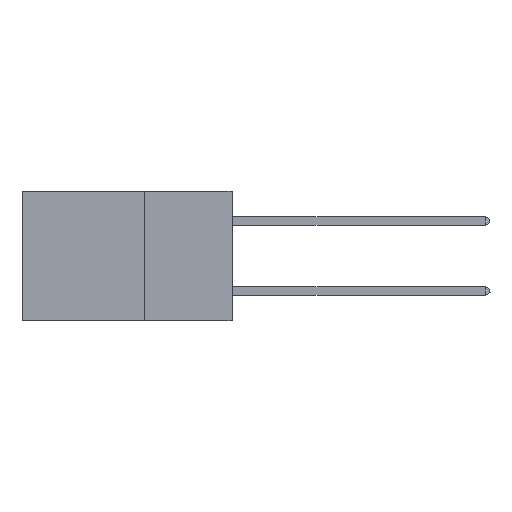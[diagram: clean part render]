
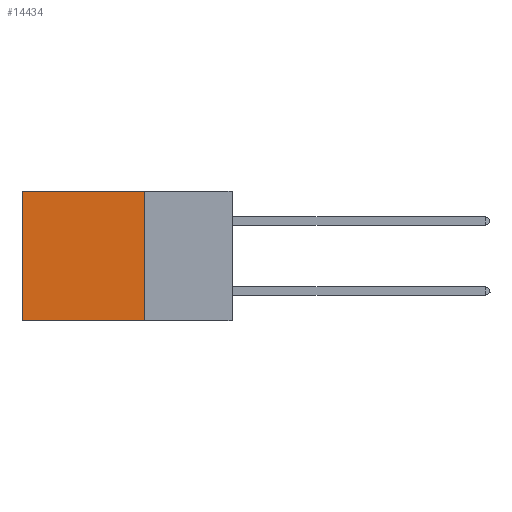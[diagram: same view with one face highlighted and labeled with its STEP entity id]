
A CAD part, left-side view. The second image highlights one B-rep face of the part: STEP entity #14434.
In plain terms, the highlighted planar face has unit normal (-1, 0, 0).
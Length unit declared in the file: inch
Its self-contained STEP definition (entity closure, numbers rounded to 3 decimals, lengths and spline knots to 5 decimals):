
#83 = AXIS2_PLACEMENT_3D ( 'NONE', #19987, #11305, #1250 ) ;
#1067 = EDGE_CURVE ( 'NONE', #20200, #18856, #13007, .T. ) ;
#1250 = DIRECTION ( 'NONE',  ( 0., 0., -1. ) ) ;
#2143 = FACE_OUTER_BOUND ( 'NONE', #9424, .T. ) ;
#2259 = CARTESIAN_POINT ( 'NONE',  ( 0.2875, 0.25, -0.37 ) ) ;
#2414 = CARTESIAN_POINT ( 'NONE',  ( 0.2875, 0.25, 0. ) ) ;
#5028 = VERTEX_POINT ( 'NONE', #18991 ) ;
#6157 = CARTESIAN_POINT ( 'NONE',  ( 0.2875, 0.25, 0. ) ) ;
#6724 = DIRECTION ( 'NONE',  ( 0., 1., 0. ) ) ;
#6842 = EDGE_CURVE ( 'NONE', #18856, #5028, #13062, .T. ) ;
#8876 = VERTEX_POINT ( 'NONE', #2259 ) ;
#9053 = CARTESIAN_POINT ( 'NONE',  ( 0.2875, 0.25, 0. ) ) ;
#9065 = VECTOR ( 'NONE', #9478, 39.37008 ) ;
#9424 = EDGE_LOOP ( 'NONE', ( #18664, #17332, #12278, #16038 ) ) ;
#9478 = DIRECTION ( 'NONE',  ( 0., 1., 0. ) ) ;
#11148 = DIRECTION ( 'NONE',  ( 0., 0., -1. ) ) ;
#11305 = DIRECTION ( 'NONE',  ( 1., 0., 0. ) ) ;
#11375 = PLANE ( 'NONE',  #83 ) ;
#11851 = LINE ( 'NONE', #6157, #14718 ) ;
#12278 = ORIENTED_EDGE ( 'NONE', *, *, #16501, .F. ) ;
#12285 = CARTESIAN_POINT ( 'NONE',  ( 0.2875, 0.6, 0. ) ) ;
#13007 = LINE ( 'NONE', #2414, #19133 ) ;
#13062 = LINE ( 'NONE', #12285, #16765 ) ;
#14042 = EDGE_CURVE ( 'NONE', #8876, #5028, #16447, .T. ) ;
#14434 = ADVANCED_FACE ( 'NONE', ( #2143 ), #11375, .F. ) ;
#14718 = VECTOR ( 'NONE', #11148, 39.37008 ) ;
#16038 = ORIENTED_EDGE ( 'NONE', *, *, #1067, .T. ) ;
#16447 = LINE ( 'NONE', #18644, #9065 ) ;
#16501 = EDGE_CURVE ( 'NONE', #20200, #8876, #11851, .T. ) ;
#16765 = VECTOR ( 'NONE', #18007, 39.37008 ) ;
#17332 = ORIENTED_EDGE ( 'NONE', *, *, #14042, .F. ) ;
#18007 = DIRECTION ( 'NONE',  ( 0., 0., -1. ) ) ;
#18644 = CARTESIAN_POINT ( 'NONE',  ( 0.2875, 0.25, -0.37 ) ) ;
#18664 = ORIENTED_EDGE ( 'NONE', *, *, #6842, .T. ) ;
#18856 = VERTEX_POINT ( 'NONE', #19051 ) ;
#18991 = CARTESIAN_POINT ( 'NONE',  ( 0.2875, 0.6, -0.37 ) ) ;
#19051 = CARTESIAN_POINT ( 'NONE',  ( 0.2875, 0.6, 0. ) ) ;
#19133 = VECTOR ( 'NONE', #6724, 39.37008 ) ;
#19987 = CARTESIAN_POINT ( 'NONE',  ( 0.2875, 0.25, 0. ) ) ;
#20200 = VERTEX_POINT ( 'NONE', #9053 ) ;
